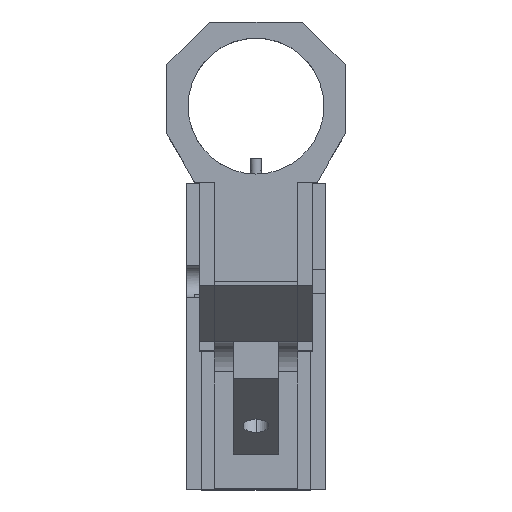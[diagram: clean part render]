
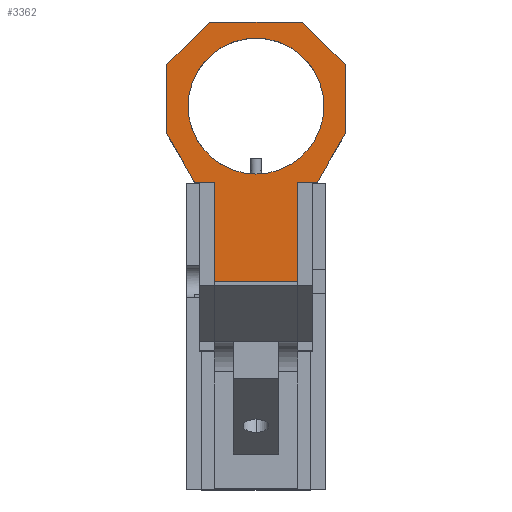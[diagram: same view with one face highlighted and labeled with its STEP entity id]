
A CAD part, top view. The second image highlights one B-rep face of the part: STEP entity #3362.
In plain terms, the highlighted planar face has unit normal (0, 0, 1).
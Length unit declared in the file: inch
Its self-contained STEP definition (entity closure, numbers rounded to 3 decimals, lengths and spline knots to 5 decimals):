
#34 = VECTOR ( 'NONE', #11055, 39.37008 ) ;
#42 = VERTEX_POINT ( 'NONE', #10071 ) ;
#70 = EDGE_CURVE ( 'NONE', #42, #741, #362, .T. ) ;
#73 = DIRECTION ( 'NONE',  ( 1., 0., 0. ) ) ;
#141 = CARTESIAN_POINT ( 'NONE',  ( -0.738, -0.22898, 0. ) ) ;
#152 = LINE ( 'NONE', #12516, #13071 ) ;
#166 = FACE_BOUND ( 'NONE', #8344, .T. ) ;
#307 = DIRECTION ( 'NONE',  ( 0.5, 0.866, 0. ) ) ;
#362 = LINE ( 'NONE', #10593, #34 ) ;
#377 = ORIENTED_EDGE ( 'NONE', *, *, #10647, .T. ) ;
#563 = ORIENTED_EDGE ( 'NONE', *, *, #10441, .T. ) ;
#593 = ORIENTED_EDGE ( 'NONE', *, *, #4409, .T. ) ;
#651 = VECTOR ( 'NONE', #8100, 39.37008 ) ;
#670 = VERTEX_POINT ( 'NONE', #5985 ) ;
#741 = VERTEX_POINT ( 'NONE', #5853 ) ;
#964 = LINE ( 'NONE', #13150, #651 ) ;
#1137 = VECTOR ( 'NONE', #3735, 39.37008 ) ;
#1141 = LINE ( 'NONE', #12982, #6271 ) ;
#1703 = VERTEX_POINT ( 'NONE', #6326 ) ;
#1738 = CIRCLE ( 'NONE', #6232, 0.5625 ) ;
#2009 = ORIENTED_EDGE ( 'NONE', *, *, #12871, .F. ) ;
#2015 = VERTEX_POINT ( 'NONE', #6813 ) ;
#2076 = DIRECTION ( 'NONE',  ( 1., 0., 0. ) ) ;
#2294 = ORIENTED_EDGE ( 'NONE', *, *, #8373, .T. ) ;
#2575 = LINE ( 'NONE', #9409, #10328 ) ;
#2672 = ORIENTED_EDGE ( 'NONE', *, *, #10234, .T. ) ;
#2680 = VERTEX_POINT ( 'NONE', #7528 ) ;
#2880 = EDGE_CURVE ( 'NONE', #2015, #670, #6278, .T. ) ;
#3194 = DIRECTION ( 'NONE',  ( 0., 0., 1. ) ) ;
#3222 = VECTOR ( 'NONE', #4162, 39.37008 ) ;
#3238 = CARTESIAN_POINT ( 'NONE',  ( -0.38445, 0.696, 0. ) ) ;
#3262 = EDGE_CURVE ( 'NONE', #670, #2680, #1141, .T. ) ;
#3348 = VECTOR ( 'NONE', #4381, 39.37008 ) ;
#3362 = ADVANCED_FACE ( 'NONE', ( #166, #5645 ), #8022, .F. ) ;
#3531 = EDGE_CURVE ( 'NONE', #9763, #8341, #9102, .T. ) ;
#3735 = DIRECTION ( 'NONE',  ( 0.5, -0.866, 0. ) ) ;
#3745 = ORIENTED_EDGE ( 'NONE', *, *, #7929, .T. ) ;
#3785 = ORIENTED_EDGE ( 'NONE', *, *, #3262, .T. ) ;
#4000 = CARTESIAN_POINT ( 'NONE',  ( 0., 0., 0. ) ) ;
#4025 = LINE ( 'NONE', #6233, #9378 ) ;
#4108 = CARTESIAN_POINT ( 'NONE',  ( -0.738, -0.22898, 0. ) ) ;
#4162 = DIRECTION ( 'NONE',  ( 0., -1., 0. ) ) ;
#4381 = DIRECTION ( 'NONE',  ( 1., 0., 0. ) ) ;
#4409 = EDGE_CURVE ( 'NONE', #1703, #10242, #9999, .T. ) ;
#4558 = EDGE_CURVE ( 'NONE', #5088, #11024, #6695, .T. ) ;
#4725 = CARTESIAN_POINT ( 'NONE',  ( 0., 0., 0. ) ) ;
#4759 = CARTESIAN_POINT ( 'NONE',  ( -0.50705, -0.629, 0. ) ) ;
#4808 = ORIENTED_EDGE ( 'NONE', *, *, #7656, .T. ) ;
#4864 = ORIENTED_EDGE ( 'NONE', *, *, #3531, .F. ) ;
#5025 = DIRECTION ( 'NONE',  ( -1., 0., 0. ) ) ;
#5088 = VERTEX_POINT ( 'NONE', #11947 ) ;
#5645 = FACE_OUTER_BOUND ( 'NONE', #12988, .T. ) ;
#5659 = ORIENTED_EDGE ( 'NONE', *, *, #70, .T. ) ;
#5746 = DIRECTION ( 'NONE',  ( 1., 0., 0. ) ) ;
#5853 = CARTESIAN_POINT ( 'NONE',  ( 0.738, 0.34245, 0. ) ) ;
#5985 = CARTESIAN_POINT ( 'NONE',  ( -0.38445, 0.696, 0. ) ) ;
#5991 = CARTESIAN_POINT ( 'NONE',  ( 0.38445, 0.696, 0. ) ) ;
#6013 = CARTESIAN_POINT ( 'NONE',  ( -0.3458, -1.448, 0. ) ) ;
#6143 = ORIENTED_EDGE ( 'NONE', *, *, #4558, .T. ) ;
#6232 = AXIS2_PLACEMENT_3D ( 'NONE', #9246, #3194, #10255 ) ;
#6233 = CARTESIAN_POINT ( 'NONE',  ( 0.3458, -1.448, 0. ) ) ;
#6271 = VECTOR ( 'NONE', #8960, 39.37008 ) ;
#6278 = LINE ( 'NONE', #3238, #10692 ) ;
#6326 = CARTESIAN_POINT ( 'NONE',  ( 0.3458, -0.629, 0. ) ) ;
#6414 = DIRECTION ( 'NONE',  ( 0., -1., 0. ) ) ;
#6505 = CARTESIAN_POINT ( 'NONE',  ( 0.3458, -1.448, 0. ) ) ;
#6615 = CARTESIAN_POINT ( 'NONE',  ( -0.5625, 0., 0. ) ) ;
#6695 = LINE ( 'NONE', #7362, #3348 ) ;
#6813 = CARTESIAN_POINT ( 'NONE',  ( 0.38445, 0.696, 0. ) ) ;
#6984 = ORIENTED_EDGE ( 'NONE', *, *, #11163, .T. ) ;
#7150 = CARTESIAN_POINT ( 'NONE',  ( 0.50705, -0.629, 0. ) ) ;
#7316 = VECTOR ( 'NONE', #2076, 39.37008 ) ;
#7362 = CARTESIAN_POINT ( 'NONE',  ( -0.3458, -0.629, 0. ) ) ;
#7528 = CARTESIAN_POINT ( 'NONE',  ( -0.738, 0.34245, 0. ) ) ;
#7656 = EDGE_CURVE ( 'NONE', #741, #2015, #11488, .T. ) ;
#7929 = EDGE_CURVE ( 'NONE', #10242, #42, #152, .T. ) ;
#8022 = PLANE ( 'NONE',  #8574 ) ;
#8073 = CARTESIAN_POINT ( 'NONE',  ( 0.5625, 0., 0. ) ) ;
#8100 = DIRECTION ( 'NONE',  ( 0., 1., 0. ) ) ;
#8341 = VERTEX_POINT ( 'NONE', #8073 ) ;
#8344 = EDGE_LOOP ( 'NONE', ( #2009, #4864 ) ) ;
#8373 = EDGE_CURVE ( 'NONE', #2680, #11680, #11309, .T. ) ;
#8471 = VECTOR ( 'NONE', #9016, 39.37008 ) ;
#8574 = AXIS2_PLACEMENT_3D ( 'NONE', #4000, #11060, #5025 ) ;
#8960 = DIRECTION ( 'NONE',  ( -0.707, -0.707, 0. ) ) ;
#9016 = DIRECTION ( 'NONE',  ( -0.707, 0.707, 0. ) ) ;
#9102 = CIRCLE ( 'NONE', #12642, 0.5625 ) ;
#9246 = CARTESIAN_POINT ( 'NONE',  ( 0., 0., 0. ) ) ;
#9291 = DIRECTION ( 'NONE',  ( -1., 0., 0. ) ) ;
#9378 = VECTOR ( 'NONE', #73, 39.37008 ) ;
#9409 = CARTESIAN_POINT ( 'NONE',  ( -0.3458, -1.448, 0. ) ) ;
#9763 = VERTEX_POINT ( 'NONE', #6615 ) ;
#9999 = LINE ( 'NONE', #7150, #7316 ) ;
#10071 = CARTESIAN_POINT ( 'NONE',  ( 0.738, -0.22898, 0. ) ) ;
#10234 = EDGE_CURVE ( 'NONE', #11680, #5088, #12278, .T. ) ;
#10242 = VERTEX_POINT ( 'NONE', #11838 ) ;
#10255 = DIRECTION ( 'NONE',  ( 1., 0., 0. ) ) ;
#10328 = VECTOR ( 'NONE', #6414, 39.37008 ) ;
#10441 = EDGE_CURVE ( 'NONE', #11795, #1703, #964, .T. ) ;
#10593 = CARTESIAN_POINT ( 'NONE',  ( 0.738, 0.34245, 0. ) ) ;
#10647 = EDGE_CURVE ( 'NONE', #11024, #11573, #2575, .T. ) ;
#10692 = VECTOR ( 'NONE', #9291, 39.37008 ) ;
#11024 = VERTEX_POINT ( 'NONE', #12038 ) ;
#11055 = DIRECTION ( 'NONE',  ( 0., 1., 0. ) ) ;
#11060 = DIRECTION ( 'NONE',  ( 0., 0., -1. ) ) ;
#11163 = EDGE_CURVE ( 'NONE', #11573, #11795, #4025, .T. ) ;
#11309 = LINE ( 'NONE', #4108, #3222 ) ;
#11488 = LINE ( 'NONE', #5991, #8471 ) ;
#11573 = VERTEX_POINT ( 'NONE', #6013 ) ;
#11680 = VERTEX_POINT ( 'NONE', #141 ) ;
#11794 = DIRECTION ( 'NONE',  ( 0., 0., 1. ) ) ;
#11795 = VERTEX_POINT ( 'NONE', #6505 ) ;
#11838 = CARTESIAN_POINT ( 'NONE',  ( 0.50705, -0.629, 0. ) ) ;
#11947 = CARTESIAN_POINT ( 'NONE',  ( -0.50705, -0.629, 0. ) ) ;
#12038 = CARTESIAN_POINT ( 'NONE',  ( -0.3458, -0.629, 0. ) ) ;
#12278 = LINE ( 'NONE', #4759, #1137 ) ;
#12516 = CARTESIAN_POINT ( 'NONE',  ( 0.738, -0.22898, 0. ) ) ;
#12642 = AXIS2_PLACEMENT_3D ( 'NONE', #4725, #11794, #5746 ) ;
#12871 = EDGE_CURVE ( 'NONE', #8341, #9763, #1738, .T. ) ;
#12982 = CARTESIAN_POINT ( 'NONE',  ( -0.738, 0.34245, 0. ) ) ;
#12983 = ORIENTED_EDGE ( 'NONE', *, *, #2880, .T. ) ;
#12988 = EDGE_LOOP ( 'NONE', ( #2294, #2672, #6143, #377, #6984, #563, #593, #3745, #5659, #4808, #12983, #3785 ) ) ;
#13071 = VECTOR ( 'NONE', #307, 39.37008 ) ;
#13150 = CARTESIAN_POINT ( 'NONE',  ( 0.3458, -0.629, 0. ) ) ;
